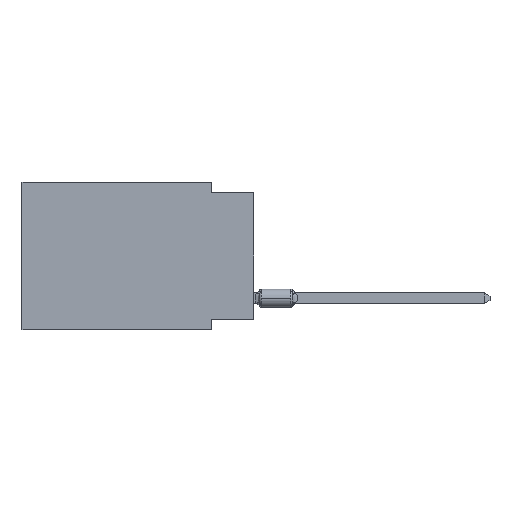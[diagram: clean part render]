
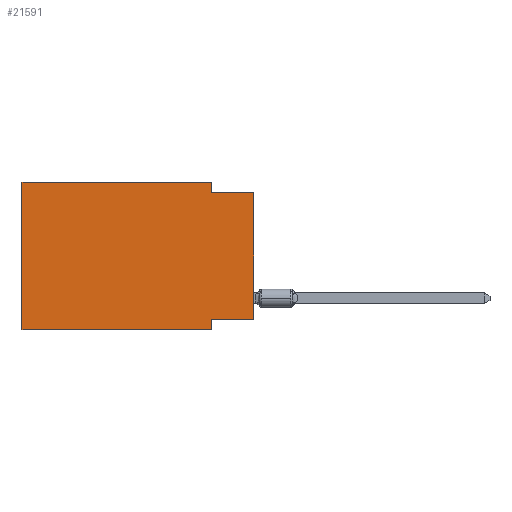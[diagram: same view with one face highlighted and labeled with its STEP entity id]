
A CAD part, left-side view. The second image highlights one B-rep face of the part: STEP entity #21591.
In plain terms, the highlighted planar face has unit normal (-1, 0, 0).
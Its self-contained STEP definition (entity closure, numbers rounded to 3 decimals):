
#1125 = CARTESIAN_POINT ( 'NONE',  ( 0., 2.54, -8.89 ) ) ;
#1175 = CARTESIAN_POINT ( 'NONE',  ( 0., 13.97, -8.89 ) ) ;
#1273 = DIRECTION ( 'NONE',  ( 0., 0., -1. ) ) ;
#1610 = ORIENTED_EDGE ( 'NONE', *, *, #4191, .F. ) ;
#1751 = VECTOR ( 'NONE', #23668, 1000. ) ;
#2831 = VECTOR ( 'NONE', #21790, 1000. ) ;
#2926 = VERTEX_POINT ( 'NONE', #23255 ) ;
#3030 = DIRECTION ( 'NONE',  ( 0., -1., 0. ) ) ;
#3209 = PLANE ( 'NONE',  #10822 ) ;
#3416 = LINE ( 'NONE', #16469, #23653 ) ;
#3769 = CARTESIAN_POINT ( 'NONE',  ( 0., 2.54, -0.635 ) ) ;
#4191 = EDGE_CURVE ( 'NONE', #15173, #15265, #5032, .T. ) ;
#4263 = CARTESIAN_POINT ( 'NONE',  ( 0., 0., -0.635 ) ) ;
#4423 = EDGE_CURVE ( 'NONE', #6640, #8671, #15158, .T. ) ;
#4598 = VECTOR ( 'NONE', #21062, 1000. ) ;
#4914 = CARTESIAN_POINT ( 'NONE',  ( 0., 13.97, 0. ) ) ;
#5032 = LINE ( 'NONE', #19753, #11304 ) ;
#6435 = CARTESIAN_POINT ( 'NONE',  ( 0., 0., -0.635 ) ) ;
#6607 = DIRECTION ( 'NONE',  ( 0., 0., -1. ) ) ;
#6640 = VERTEX_POINT ( 'NONE', #1175 ) ;
#7054 = DIRECTION ( 'NONE',  ( 0., 0., 1. ) ) ;
#8039 = CARTESIAN_POINT ( 'NONE',  ( 0., 13.97, -8.89 ) ) ;
#8671 = VERTEX_POINT ( 'NONE', #1125 ) ;
#8677 = CARTESIAN_POINT ( 'NONE',  ( 0., 2.54, -8.89 ) ) ;
#8954 = CARTESIAN_POINT ( 'NONE',  ( 0., 13.97, 0. ) ) ;
#9367 = EDGE_CURVE ( 'NONE', #21478, #15173, #12331, .T. ) ;
#9829 = VERTEX_POINT ( 'NONE', #12665 ) ;
#10184 = ORIENTED_EDGE ( 'NONE', *, *, #19057, .F. ) ;
#10207 = LINE ( 'NONE', #12019, #4598 ) ;
#10433 = ORIENTED_EDGE ( 'NONE', *, *, #13080, .F. ) ;
#10822 = AXIS2_PLACEMENT_3D ( 'NONE', #4914, #12291, #1273 ) ;
#11304 = VECTOR ( 'NONE', #6607, 1000. ) ;
#12019 = CARTESIAN_POINT ( 'NONE',  ( 0., 0., -8.255 ) ) ;
#12291 = DIRECTION ( 'NONE',  ( 1., 0., 0. ) ) ;
#12296 = LINE ( 'NONE', #8677, #20237 ) ;
#12331 = LINE ( 'NONE', #8954, #1751 ) ;
#12665 = CARTESIAN_POINT ( 'NONE',  ( 0., 2.54, -8.255 ) ) ;
#13080 = EDGE_CURVE ( 'NONE', #6640, #21478, #3416, .T. ) ;
#13788 = EDGE_LOOP ( 'NONE', ( #22363, #10184, #1610, #21476, #10433, #19515, #19894, #18993 ) ) ;
#13847 = CARTESIAN_POINT ( 'NONE',  ( 0., 0., 0. ) ) ;
#13922 = LINE ( 'NONE', #6435, #22282 ) ;
#14318 = EDGE_CURVE ( 'NONE', #9829, #8671, #12296, .T. ) ;
#14690 = EDGE_CURVE ( 'NONE', #2926, #23400, #15531, .T. ) ;
#15158 = LINE ( 'NONE', #8039, #17065 ) ;
#15173 = VERTEX_POINT ( 'NONE', #23335 ) ;
#15265 = VERTEX_POINT ( 'NONE', #3769 ) ;
#15531 = LINE ( 'NONE', #13847, #2831 ) ;
#16469 = CARTESIAN_POINT ( 'NONE',  ( 0., 13.97, 0. ) ) ;
#17065 = VECTOR ( 'NONE', #18891, 1000. ) ;
#18891 = DIRECTION ( 'NONE',  ( 0., -1., 0. ) ) ;
#18993 = ORIENTED_EDGE ( 'NONE', *, *, #20267, .F. ) ;
#19057 = EDGE_CURVE ( 'NONE', #15265, #23400, #13922, .T. ) ;
#19515 = ORIENTED_EDGE ( 'NONE', *, *, #4423, .T. ) ;
#19753 = CARTESIAN_POINT ( 'NONE',  ( 0., 2.54, 0. ) ) ;
#19887 = DIRECTION ( 'NONE',  ( 0., 0., -1. ) ) ;
#19894 = ORIENTED_EDGE ( 'NONE', *, *, #14318, .F. ) ;
#20237 = VECTOR ( 'NONE', #19887, 1000. ) ;
#20267 = EDGE_CURVE ( 'NONE', #2926, #9829, #10207, .T. ) ;
#21062 = DIRECTION ( 'NONE',  ( 0., 1., 0. ) ) ;
#21446 = FACE_OUTER_BOUND ( 'NONE', #13788, .T. ) ;
#21476 = ORIENTED_EDGE ( 'NONE', *, *, #9367, .F. ) ;
#21478 = VERTEX_POINT ( 'NONE', #22907 ) ;
#21591 = ADVANCED_FACE ( 'NONE', ( #21446 ), #3209, .F. ) ;
#21790 = DIRECTION ( 'NONE',  ( 0., 0., 1. ) ) ;
#22282 = VECTOR ( 'NONE', #3030, 1000. ) ;
#22363 = ORIENTED_EDGE ( 'NONE', *, *, #14690, .T. ) ;
#22907 = CARTESIAN_POINT ( 'NONE',  ( 0., 13.97, 0. ) ) ;
#23255 = CARTESIAN_POINT ( 'NONE',  ( 0., 0., -8.255 ) ) ;
#23335 = CARTESIAN_POINT ( 'NONE',  ( 0., 2.54, 0. ) ) ;
#23400 = VERTEX_POINT ( 'NONE', #4263 ) ;
#23653 = VECTOR ( 'NONE', #7054, 1000. ) ;
#23668 = DIRECTION ( 'NONE',  ( 0., -1., 0. ) ) ;
